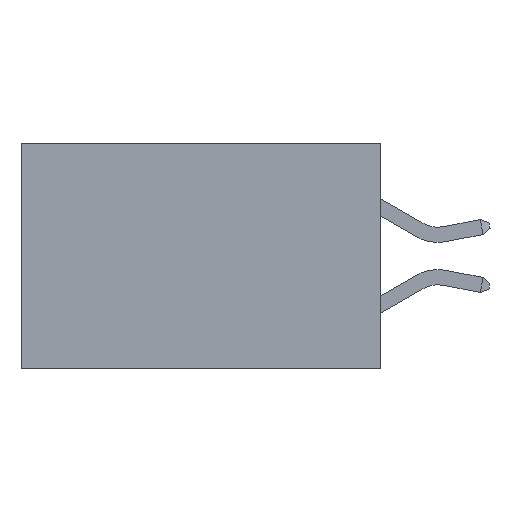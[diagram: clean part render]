
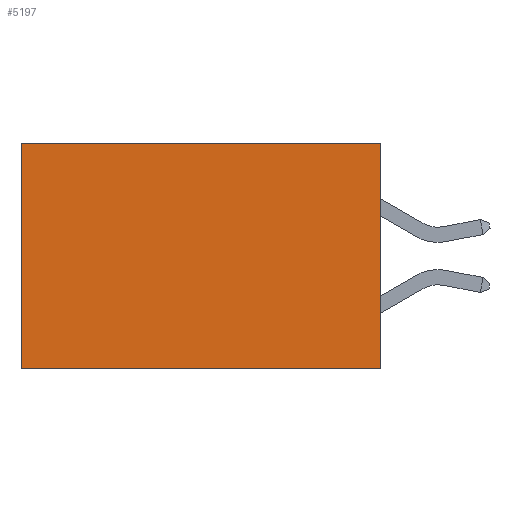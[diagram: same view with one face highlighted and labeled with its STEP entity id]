
A CAD part, left-side view. The second image highlights one B-rep face of the part: STEP entity #5197.
In plain terms, the highlighted planar face has unit normal (-1, 0, 0).
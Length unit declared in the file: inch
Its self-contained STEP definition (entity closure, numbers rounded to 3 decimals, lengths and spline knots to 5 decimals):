
#1090 = CARTESIAN_POINT ( 'NONE',  ( 0.277, 0., -0.37 ) ) ;
#1563 = DIRECTION ( 'NONE',  ( 0., 0., -1. ) ) ;
#1658 = LINE ( 'NONE', #17919, #6893 ) ;
#1766 = VECTOR ( 'NONE', #1563, 39.37008 ) ;
#2529 = EDGE_CURVE ( 'NONE', #15704, #11961, #25800, .T. ) ;
#5142 = FACE_OUTER_BOUND ( 'NONE', #7733, .T. ) ;
#5197 = ADVANCED_FACE ( 'NONE', ( #5142 ), #16922, .F. ) ;
#5852 = ORIENTED_EDGE ( 'NONE', *, *, #2529, .F. ) ;
#6893 = VECTOR ( 'NONE', #18014, 39.37008 ) ;
#7733 = EDGE_LOOP ( 'NONE', ( #11008, #5852, #11556, #26258 ) ) ;
#8019 = CARTESIAN_POINT ( 'NONE',  ( 0.277, 0., -0.37 ) ) ;
#8246 = CARTESIAN_POINT ( 'NONE',  ( 0.277, 0.59, -0.37 ) ) ;
#9628 = VERTEX_POINT ( 'NONE', #17238 ) ;
#11008 = ORIENTED_EDGE ( 'NONE', *, *, #25577, .T. ) ;
#11556 = ORIENTED_EDGE ( 'NONE', *, *, #12651, .F. ) ;
#11805 = VECTOR ( 'NONE', #17596, 39.37008 ) ;
#11961 = VERTEX_POINT ( 'NONE', #8246 ) ;
#12113 = VERTEX_POINT ( 'NONE', #12967 ) ;
#12574 = CARTESIAN_POINT ( 'NONE',  ( 0.277, 0., -0.37 ) ) ;
#12651 = EDGE_CURVE ( 'NONE', #9628, #15704, #19277, .T. ) ;
#12967 = CARTESIAN_POINT ( 'NONE',  ( 0.277, 0.59, 0. ) ) ;
#15390 = CARTESIAN_POINT ( 'NONE',  ( 0.277, 0.59, -0.37 ) ) ;
#15704 = VERTEX_POINT ( 'NONE', #1090 ) ;
#16771 = DIRECTION ( 'NONE',  ( 0., 0., -1. ) ) ;
#16889 = DIRECTION ( 'NONE',  ( 1., 0., 0. ) ) ;
#16922 = PLANE ( 'NONE',  #21864 ) ;
#17073 = CARTESIAN_POINT ( 'NONE',  ( 0.277, 0., -0.37 ) ) ;
#17238 = CARTESIAN_POINT ( 'NONE',  ( 0.277, 0., 0. ) ) ;
#17596 = DIRECTION ( 'NONE',  ( 0., 0., -1. ) ) ;
#17919 = CARTESIAN_POINT ( 'NONE',  ( 0.277, 0., 0. ) ) ;
#18014 = DIRECTION ( 'NONE',  ( 0., 1., 0. ) ) ;
#18274 = LINE ( 'NONE', #15390, #11805 ) ;
#19277 = LINE ( 'NONE', #12574, #1766 ) ;
#20850 = DIRECTION ( 'NONE',  ( 0., 1., 0. ) ) ;
#21864 = AXIS2_PLACEMENT_3D ( 'NONE', #17073, #16889, #16771 ) ;
#25114 = VECTOR ( 'NONE', #20850, 39.37008 ) ;
#25577 = EDGE_CURVE ( 'NONE', #12113, #11961, #18274, .T. ) ;
#25800 = LINE ( 'NONE', #8019, #25114 ) ;
#26258 = ORIENTED_EDGE ( 'NONE', *, *, #27529, .T. ) ;
#27529 = EDGE_CURVE ( 'NONE', #9628, #12113, #1658, .T. ) ;
